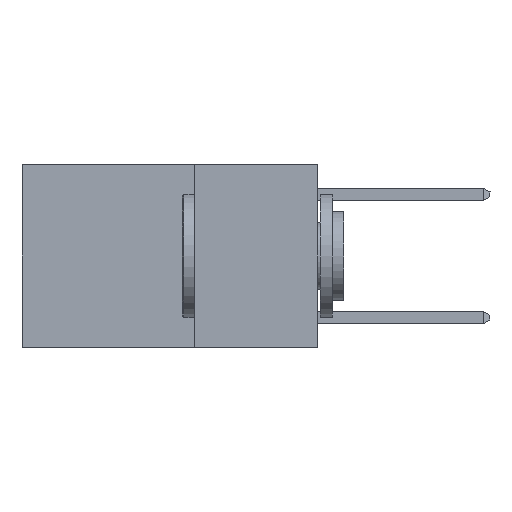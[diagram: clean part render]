
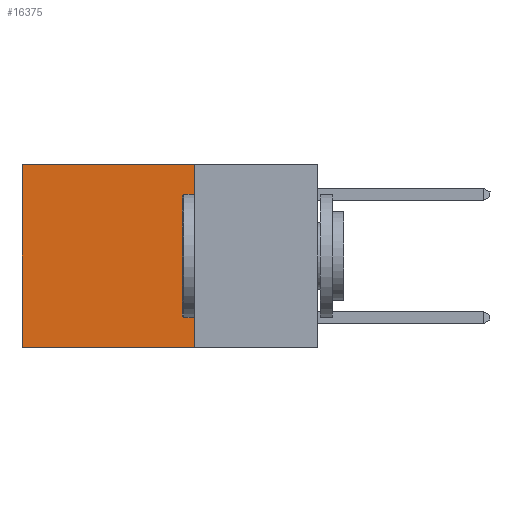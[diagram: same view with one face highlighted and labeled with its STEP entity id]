
A CAD part, left-side view. The second image highlights one B-rep face of the part: STEP entity #16375.
In plain terms, the highlighted planar face has unit normal (-1, 0, 0).
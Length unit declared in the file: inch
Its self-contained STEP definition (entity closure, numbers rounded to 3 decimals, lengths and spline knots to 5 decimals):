
#108 = VECTOR ( 'NONE', #16817, 39.37008 ) ;
#1184 = CARTESIAN_POINT ( 'NONE',  ( 0.2625, 0.6, 0. ) ) ;
#2678 = CARTESIAN_POINT ( 'NONE',  ( 0.2625, 0.25, -0.37 ) ) ;
#3039 = DIRECTION ( 'NONE',  ( 0., 0., -1. ) ) ;
#3138 = VECTOR ( 'NONE', #13114, 39.37008 ) ;
#3298 = CARTESIAN_POINT ( 'NONE',  ( 0.2625, 0.6, -0.37 ) ) ;
#3739 = CARTESIAN_POINT ( 'NONE',  ( 0.2625, 0.25, 0. ) ) ;
#3818 = VERTEX_POINT ( 'NONE', #1184 ) ;
#3933 = VECTOR ( 'NONE', #13886, 39.37008 ) ;
#4898 = CARTESIAN_POINT ( 'NONE',  ( 0.2625, 0.6, 0. ) ) ;
#4910 = EDGE_CURVE ( 'NONE', #17354, #6816, #18566, .T. ) ;
#5128 = ORIENTED_EDGE ( 'NONE', *, *, #4910, .F. ) ;
#5199 = DIRECTION ( 'NONE',  ( 0., 0., -1. ) ) ;
#5857 = ORIENTED_EDGE ( 'NONE', *, *, #15539, .T. ) ;
#6417 = EDGE_LOOP ( 'NONE', ( #5857, #8251, #5128, #8989 ) ) ;
#6816 = VERTEX_POINT ( 'NONE', #8832 ) ;
#8130 = EDGE_CURVE ( 'NONE', #6816, #15507, #10611, .T. ) ;
#8251 = ORIENTED_EDGE ( 'NONE', *, *, #8130, .F. ) ;
#8832 = CARTESIAN_POINT ( 'NONE',  ( 0.2625, 0.25, -0.37 ) ) ;
#8989 = ORIENTED_EDGE ( 'NONE', *, *, #11773, .T. ) ;
#9414 = FACE_OUTER_BOUND ( 'NONE', #6417, .T. ) ;
#10611 = LINE ( 'NONE', #2678, #3138 ) ;
#11773 = EDGE_CURVE ( 'NONE', #17354, #3818, #15795, .T. ) ;
#12377 = CARTESIAN_POINT ( 'NONE',  ( 0.2625, 0.25, 0. ) ) ;
#12493 = LINE ( 'NONE', #4898, #108 ) ;
#12600 = PLANE ( 'NONE',  #16309 ) ;
#13114 = DIRECTION ( 'NONE',  ( 0., 1., 0. ) ) ;
#13886 = DIRECTION ( 'NONE',  ( 0., 1., 0. ) ) ;
#14156 = DIRECTION ( 'NONE',  ( 1., 0., 0. ) ) ;
#14617 = VECTOR ( 'NONE', #3039, 39.37008 ) ;
#15507 = VERTEX_POINT ( 'NONE', #3298 ) ;
#15539 = EDGE_CURVE ( 'NONE', #3818, #15507, #12493, .T. ) ;
#15795 = LINE ( 'NONE', #12377, #3933 ) ;
#16309 = AXIS2_PLACEMENT_3D ( 'NONE', #3739, #14156, #5199 ) ;
#16375 = ADVANCED_FACE ( 'NONE', ( #9414 ), #12600, .F. ) ;
#16817 = DIRECTION ( 'NONE',  ( 0., 0., -1. ) ) ;
#17317 = CARTESIAN_POINT ( 'NONE',  ( 0.2625, 0.25, 0. ) ) ;
#17354 = VERTEX_POINT ( 'NONE', #17317 ) ;
#17865 = CARTESIAN_POINT ( 'NONE',  ( 0.2625, 0.25, 0. ) ) ;
#18566 = LINE ( 'NONE', #17865, #14617 ) ;
